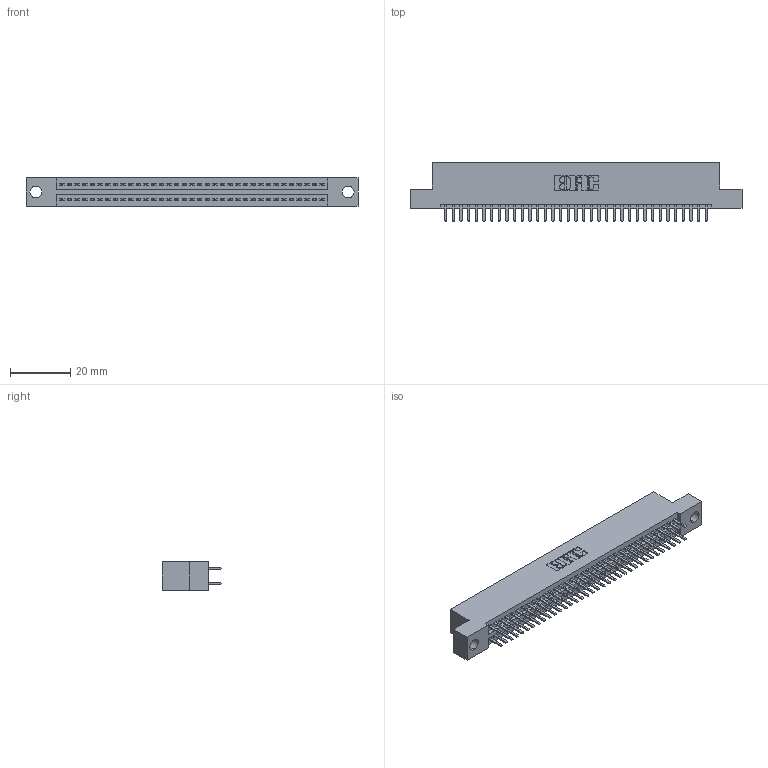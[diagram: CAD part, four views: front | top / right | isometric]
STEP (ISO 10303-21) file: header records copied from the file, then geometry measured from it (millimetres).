
FILE_DESCRIPTION (( 'STEP AP203' ), '1' );
FILE_NAME ('345-070-520-204.STEP', '2018-09-30T22:15:07', ( '' ), ( '' ), 'SwSTEP 2.0', 'SolidWorks 2016', '' );
FILE_SCHEMA (( 'CONFIG_CONTROL_DESIGN' ));
Length unit declared in the file: inch
Products named in the file (3): 345-292-001_345-293-120; 345-070-520-204; 345 Part_Flush Mounting Lugs - 0.156 Dia-TH
Assembly tree (71 placements, depth 2):
  345-070-520-204
    345 Part_Flush Mounting Lugs - 0.156 Dia-TH
    345-292-001_345-293-120  x70
Bounding box: 110.11 x 19.68 x 9.4 mm (x, y, z)
Volume: 10512.5 mm3; surface area: 15153.4 mm2
Topology: 71 solids, 71 shells, 3906 faces, 11331 edges, 7366 vertices
Faces by surface type: plane 2530, cylinder 1376
Entity records: 28521 total; most frequent: CARTESIAN_POINT 4800, ORIENTED_EDGE 4722, DIRECTION 4229, EDGE_CURVE 2361, VECTOR 2085, LINE 2085, VERTEX_POINT 1570, AXIS2_PLACEMENT_3D 1072
